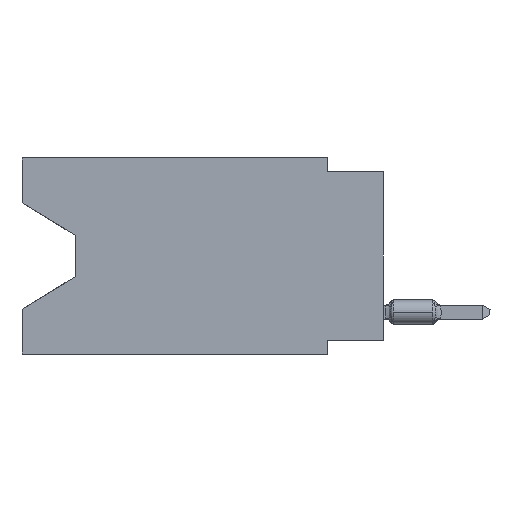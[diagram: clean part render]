
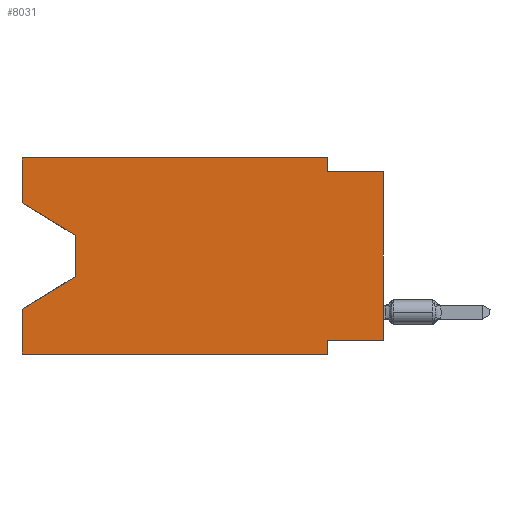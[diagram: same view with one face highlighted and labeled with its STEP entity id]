
A CAD part, left-side view. The second image highlights one B-rep face of the part: STEP entity #8031.
In plain terms, the highlighted planar face has unit normal (-1, 0, 0).
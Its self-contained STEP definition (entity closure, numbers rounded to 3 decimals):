
#445 = VECTOR ( 'NONE', #10744, 1000. ) ;
#713 = DIRECTION ( 'NONE',  ( 0., 0., -1. ) ) ;
#1180 = VERTEX_POINT ( 'NONE', #16803 ) ;
#1296 = CARTESIAN_POINT ( 'NONE',  ( 0., 0., -0.635 ) ) ;
#1359 = EDGE_CURVE ( 'NONE', #9843, #1180, #7876, .T. ) ;
#1420 = LINE ( 'NONE', #7786, #6760 ) ;
#1541 = VERTEX_POINT ( 'NONE', #1296 ) ;
#1819 = CARTESIAN_POINT ( 'NONE',  ( 0., 16.383, 0. ) ) ;
#2205 = VECTOR ( 'NONE', #17487, 1000. ) ;
#2483 = CARTESIAN_POINT ( 'NONE',  ( 0., 0., -8.255 ) ) ;
#3395 = ORIENTED_EDGE ( 'NONE', *, *, #16918, .T. ) ;
#3721 = ORIENTED_EDGE ( 'NONE', *, *, #17800, .T. ) ;
#3862 = LINE ( 'NONE', #17391, #12689 ) ;
#4835 = VERTEX_POINT ( 'NONE', #19163 ) ;
#5268 = EDGE_CURVE ( 'NONE', #1180, #18668, #1420, .T. ) ;
#5369 = VECTOR ( 'NONE', #14681, 1000. ) ;
#5853 = DIRECTION ( 'NONE',  ( 0., 0., 1. ) ) ;
#5863 = LINE ( 'NONE', #8665, #8264 ) ;
#6054 = EDGE_CURVE ( 'NONE', #18668, #1541, #17399, .T. ) ;
#6126 = ORIENTED_EDGE ( 'NONE', *, *, #6981, .T. ) ;
#6316 = EDGE_CURVE ( 'NONE', #15246, #8638, #9322, .T. ) ;
#6347 = AXIS2_PLACEMENT_3D ( 'NONE', #1819, #18724, #713 ) ;
#6616 = CARTESIAN_POINT ( 'NONE',  ( 0., 16.383, -2.038 ) ) ;
#6760 = VECTOR ( 'NONE', #16526, 1000. ) ;
#6981 = EDGE_CURVE ( 'NONE', #10565, #15679, #17204, .T. ) ;
#7250 = EDGE_CURVE ( 'NONE', #18745, #9843, #7446, .T. ) ;
#7446 = LINE ( 'NONE', #10443, #12795 ) ;
#7700 = ORIENTED_EDGE ( 'NONE', *, *, #5268, .F. ) ;
#7786 = CARTESIAN_POINT ( 'NONE',  ( 0., 2.54, 0. ) ) ;
#7808 = CARTESIAN_POINT ( 'NONE',  ( 0., 2.54, -0.635 ) ) ;
#7816 = VECTOR ( 'NONE', #9772, 1000. ) ;
#7840 = CARTESIAN_POINT ( 'NONE',  ( 0., 2.54, -8.89 ) ) ;
#7876 = LINE ( 'NONE', #18715, #7816 ) ;
#8031 = ADVANCED_FACE ( 'NONE', ( #12559 ), #12858, .F. ) ;
#8205 = CARTESIAN_POINT ( 'NONE',  ( 0., 0., -8.255 ) ) ;
#8264 = VECTOR ( 'NONE', #14751, 1000. ) ;
#8386 = VECTOR ( 'NONE', #13132, 1000. ) ;
#8638 = VERTEX_POINT ( 'NONE', #12791 ) ;
#8665 = CARTESIAN_POINT ( 'NONE',  ( 0., 16.383, -2.038 ) ) ;
#9322 = LINE ( 'NONE', #7840, #17272 ) ;
#9536 = CARTESIAN_POINT ( 'NONE',  ( 0., 16.383, 0. ) ) ;
#9772 = DIRECTION ( 'NONE',  ( 0., -1., 0. ) ) ;
#9843 = VERTEX_POINT ( 'NONE', #11229 ) ;
#9845 = DIRECTION ( 'NONE',  ( 0., 0., 1. ) ) ;
#10295 = ORIENTED_EDGE ( 'NONE', *, *, #7250, .F. ) ;
#10381 = LINE ( 'NONE', #12052, #5369 ) ;
#10443 = CARTESIAN_POINT ( 'NONE',  ( 0., 16.383, 0. ) ) ;
#10565 = VERTEX_POINT ( 'NONE', #13843 ) ;
#10744 = DIRECTION ( 'NONE',  ( 0., 0.855, -0.519 ) ) ;
#11123 = CARTESIAN_POINT ( 'NONE',  ( 0., 2.54, -8.255 ) ) ;
#11229 = CARTESIAN_POINT ( 'NONE',  ( 0., 16.383, 0. ) ) ;
#11508 = VECTOR ( 'NONE', #14438, 1000. ) ;
#11836 = CARTESIAN_POINT ( 'NONE',  ( 0., 13.97, -5.385 ) ) ;
#12030 = LINE ( 'NONE', #12430, #445 ) ;
#12052 = CARTESIAN_POINT ( 'NONE',  ( 0., 16.383, -8.89 ) ) ;
#12430 = CARTESIAN_POINT ( 'NONE',  ( 0., 13.97, -5.385 ) ) ;
#12559 = FACE_OUTER_BOUND ( 'NONE', #15474, .T. ) ;
#12689 = VECTOR ( 'NONE', #9845, 1000. ) ;
#12791 = CARTESIAN_POINT ( 'NONE',  ( 0., 2.54, -8.89 ) ) ;
#12795 = VECTOR ( 'NONE', #5853, 1000. ) ;
#12824 = ORIENTED_EDGE ( 'NONE', *, *, #15200, .F. ) ;
#12858 = PLANE ( 'NONE',  #6347 ) ;
#13132 = DIRECTION ( 'NONE',  ( 0., -1., 0. ) ) ;
#13706 = ORIENTED_EDGE ( 'NONE', *, *, #6054, .F. ) ;
#13843 = CARTESIAN_POINT ( 'NONE',  ( 0., 13.97, -3.505 ) ) ;
#14024 = VERTEX_POINT ( 'NONE', #8205 ) ;
#14438 = DIRECTION ( 'NONE',  ( 0., 0., -1. ) ) ;
#14639 = CARTESIAN_POINT ( 'NONE',  ( 0., 0., -0.635 ) ) ;
#14669 = EDGE_CURVE ( 'NONE', #15679, #4835, #12030, .T. ) ;
#14681 = DIRECTION ( 'NONE',  ( 0., -1., 0. ) ) ;
#14751 = DIRECTION ( 'NONE',  ( 0., -0.855, -0.519 ) ) ;
#15160 = ORIENTED_EDGE ( 'NONE', *, *, #14669, .T. ) ;
#15200 = EDGE_CURVE ( 'NONE', #18928, #4835, #19035, .T. ) ;
#15246 = VERTEX_POINT ( 'NONE', #11123 ) ;
#15417 = ORIENTED_EDGE ( 'NONE', *, *, #1359, .F. ) ;
#15474 = EDGE_LOOP ( 'NONE', ( #19266, #6126, #15160, #12824, #3721, #19504, #18482, #3395, #13706, #7700, #15417, #10295 ) ) ;
#15679 = VERTEX_POINT ( 'NONE', #11836 ) ;
#15696 = DIRECTION ( 'NONE',  ( 0., 0., 1. ) ) ;
#15769 = CARTESIAN_POINT ( 'NONE',  ( 0., 16.383, -8.89 ) ) ;
#16091 = LINE ( 'NONE', #2483, #2205 ) ;
#16526 = DIRECTION ( 'NONE',  ( 0., 0., -1. ) ) ;
#16803 = CARTESIAN_POINT ( 'NONE',  ( 0., 2.54, 0. ) ) ;
#16918 = EDGE_CURVE ( 'NONE', #14024, #1541, #3862, .T. ) ;
#16941 = EDGE_CURVE ( 'NONE', #14024, #15246, #16091, .T. ) ;
#17204 = LINE ( 'NONE', #18508, #11508 ) ;
#17272 = VECTOR ( 'NONE', #18685, 1000. ) ;
#17391 = CARTESIAN_POINT ( 'NONE',  ( 0., 0., 0. ) ) ;
#17399 = LINE ( 'NONE', #14639, #8386 ) ;
#17487 = DIRECTION ( 'NONE',  ( 0., 1., 0. ) ) ;
#17800 = EDGE_CURVE ( 'NONE', #18928, #8638, #10381, .T. ) ;
#18263 = EDGE_CURVE ( 'NONE', #18745, #10565, #5863, .T. ) ;
#18482 = ORIENTED_EDGE ( 'NONE', *, *, #16941, .F. ) ;
#18508 = CARTESIAN_POINT ( 'NONE',  ( 0., 13.97, -3.505 ) ) ;
#18668 = VERTEX_POINT ( 'NONE', #7808 ) ;
#18685 = DIRECTION ( 'NONE',  ( 0., 0., -1. ) ) ;
#18715 = CARTESIAN_POINT ( 'NONE',  ( 0., 16.383, 0. ) ) ;
#18724 = DIRECTION ( 'NONE',  ( 1., 0., 0. ) ) ;
#18745 = VERTEX_POINT ( 'NONE', #6616 ) ;
#18799 = VECTOR ( 'NONE', #15696, 1000. ) ;
#18928 = VERTEX_POINT ( 'NONE', #15769 ) ;
#19035 = LINE ( 'NONE', #9536, #18799 ) ;
#19163 = CARTESIAN_POINT ( 'NONE',  ( 0., 16.383, -6.852 ) ) ;
#19266 = ORIENTED_EDGE ( 'NONE', *, *, #18263, .T. ) ;
#19504 = ORIENTED_EDGE ( 'NONE', *, *, #6316, .F. ) ;
